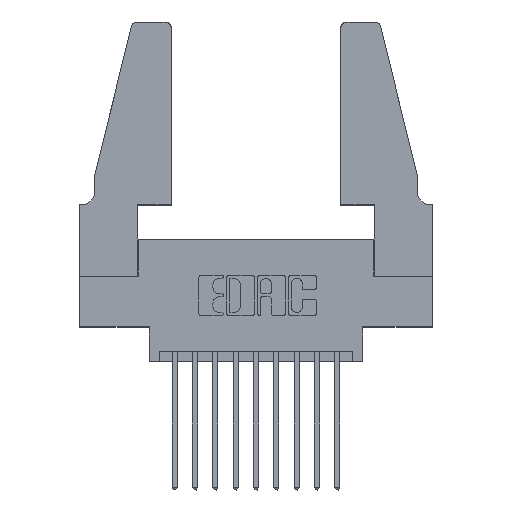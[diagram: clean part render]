
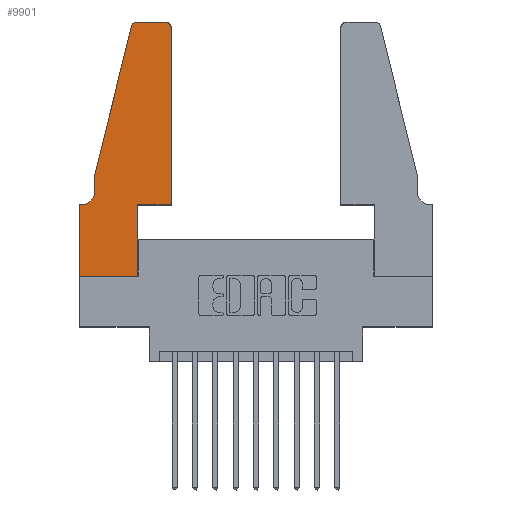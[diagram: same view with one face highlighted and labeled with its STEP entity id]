
A CAD part, top view. The second image highlights one B-rep face of the part: STEP entity #9901.
In plain terms, the highlighted planar face has unit normal (0, 0, 1).
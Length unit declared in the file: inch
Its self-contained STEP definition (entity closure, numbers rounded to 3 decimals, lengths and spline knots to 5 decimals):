
#49 = EDGE_CURVE ( 'NONE', #7841, #9602, #7819, .T. ) ;
#59 = DIRECTION ( 'NONE',  ( -1., 0., 0. ) ) ;
#118 = CARTESIAN_POINT ( 'NONE',  ( 0.2865, 0.35, 0.37 ) ) ;
#161 = DIRECTION ( 'NONE',  ( 0., 1., 0. ) ) ;
#573 = CARTESIAN_POINT ( 'NONE',  ( 0.2865, 0.35, 0.37 ) ) ;
#742 = ORIENTED_EDGE ( 'NONE', *, *, #4941, .T. ) ;
#955 = LINE ( 'NONE', #10663, #5234 ) ;
#1137 = DIRECTION ( 'NONE',  ( -1., 0., 0. ) ) ;
#1198 = VERTEX_POINT ( 'NONE', #6475 ) ;
#1309 = CARTESIAN_POINT ( 'NONE',  ( 0.0755, 0.5, 0.37 ) ) ;
#1310 = DIRECTION ( 'NONE',  ( -1., 0., 0. ) ) ;
#1605 = EDGE_LOOP ( 'NONE', ( #12128, #742, #8746, #7917, #6020, #7271, #11138, #9298, #1610, #8991, #12434, #9938 ) ) ;
#1610 = ORIENTED_EDGE ( 'NONE', *, *, #8606, .T. ) ;
#1633 = DIRECTION ( 'NONE',  ( 1., 0., 0. ) ) ;
#2351 = CARTESIAN_POINT ( 'NONE',  ( 0.4205, 1.22, 0.37 ) ) ;
#3048 = LINE ( 'NONE', #11679, #7726 ) ;
#3116 = EDGE_CURVE ( 'NONE', #10071, #5017, #7274, .T. ) ;
#3377 = CARTESIAN_POINT ( 'NONE',  ( 0.0055, 0.42, 0.37 ) ) ;
#3413 = CARTESIAN_POINT ( 'NONE',  ( 0.284, 1.22, 0.37 ) ) ;
#3847 = CARTESIAN_POINT ( 'NONE',  ( 0.4205, 1.25, 0.37 ) ) ;
#4272 = DIRECTION ( 'NONE',  ( 0., -1., 0. ) ) ;
#4383 = DIRECTION ( 'NONE',  ( 0., -1., 0. ) ) ;
#4542 = EDGE_CURVE ( 'NONE', #12759, #10071, #8392, .T. ) ;
#4570 = DIRECTION ( 'NONE',  ( 1., 0., 0. ) ) ;
#4941 = EDGE_CURVE ( 'NONE', #1198, #10855, #8474, .T. ) ;
#4995 = CARTESIAN_POINT ( 'NONE',  ( 0.4505, 1.22, 0.37 ) ) ;
#5017 = VERTEX_POINT ( 'NONE', #11174 ) ;
#5051 = VECTOR ( 'NONE', #4383, 39.37008 ) ;
#5080 = DIRECTION ( 'NONE',  ( 1., 0., 0. ) ) ;
#5096 = VERTEX_POINT ( 'NONE', #13667 ) ;
#5234 = VECTOR ( 'NONE', #4272, 39.37008 ) ;
#5282 = CARTESIAN_POINT ( 'NONE',  ( 0.0755, 0.35, 0.37 ) ) ;
#5436 = AXIS2_PLACEMENT_3D ( 'NONE', #3413, #5685, #6741 ) ;
#5554 = AXIS2_PLACEMENT_3D ( 'NONE', #11178, #7035, #1633 ) ;
#5685 = DIRECTION ( 'NONE',  ( 0., 0., 1. ) ) ;
#5698 = VECTOR ( 'NONE', #161, 39.37008 ) ;
#6020 = ORIENTED_EDGE ( 'NONE', *, *, #4542, .T. ) ;
#6046 = VERTEX_POINT ( 'NONE', #8072 ) ;
#6053 = LINE ( 'NONE', #118, #5698 ) ;
#6338 = FACE_OUTER_BOUND ( 'NONE', #1605, .T. ) ;
#6475 = CARTESIAN_POINT ( 'NONE',  ( 0.284, 1.25, 0.37 ) ) ;
#6741 = DIRECTION ( 'NONE',  ( 1., 0., 0. ) ) ;
#6918 = VECTOR ( 'NONE', #7499, 39.37008 ) ;
#6952 = EDGE_CURVE ( 'NONE', #6046, #5096, #13807, .T. ) ;
#7035 = DIRECTION ( 'NONE',  ( 0., 0., 1. ) ) ;
#7271 = ORIENTED_EDGE ( 'NONE', *, *, #3116, .T. ) ;
#7274 = LINE ( 'NONE', #5282, #12598 ) ;
#7499 = DIRECTION ( 'NONE',  ( -0.239, -0.971, 0. ) ) ;
#7674 = CARTESIAN_POINT ( 'NONE',  ( 0.0755, 0.42, 0.37 ) ) ;
#7726 = VECTOR ( 'NONE', #59, 39.37008 ) ;
#7819 = CIRCLE ( 'NONE', #7831, 0.03 ) ;
#7831 = AXIS2_PLACEMENT_3D ( 'NONE', #2351, #11991, #4570 ) ;
#7841 = VERTEX_POINT ( 'NONE', #4995 ) ;
#7917 = ORIENTED_EDGE ( 'NONE', *, *, #11423, .T. ) ;
#8072 = CARTESIAN_POINT ( 'NONE',  ( 0., 0., 0.37 ) ) ;
#8118 = VECTOR ( 'NONE', #12546, 39.37008 ) ;
#8348 = VECTOR ( 'NONE', #5080, 39.37008 ) ;
#8385 = EDGE_CURVE ( 'NONE', #8601, #7841, #9073, .T. ) ;
#8392 = CIRCLE ( 'NONE', #10286, 0.07 ) ;
#8396 = DIRECTION ( 'NONE',  ( 0., 1., 0. ) ) ;
#8474 = CIRCLE ( 'NONE', #5436, 0.03 ) ;
#8567 = EDGE_CURVE ( 'NONE', #5017, #6046, #12408, .T. ) ;
#8601 = VERTEX_POINT ( 'NONE', #10777 ) ;
#8606 = EDGE_CURVE ( 'NONE', #5096, #9912, #6053, .T. ) ;
#8746 = ORIENTED_EDGE ( 'NONE', *, *, #12713, .T. ) ;
#8991 = ORIENTED_EDGE ( 'NONE', *, *, #11323, .T. ) ;
#9073 = LINE ( 'NONE', #13731, #10068 ) ;
#9298 = ORIENTED_EDGE ( 'NONE', *, *, #6952, .T. ) ;
#9541 = CARTESIAN_POINT ( 'NONE',  ( 0.0755, 0.5, 0.37 ) ) ;
#9602 = VERTEX_POINT ( 'NONE', #3847 ) ;
#9901 = ADVANCED_FACE ( 'NONE', ( #6338 ), #13437, .T. ) ;
#9912 = VERTEX_POINT ( 'NONE', #573 ) ;
#9938 = ORIENTED_EDGE ( 'NONE', *, *, #49, .T. ) ;
#10068 = VECTOR ( 'NONE', #8396, 39.37008 ) ;
#10071 = VERTEX_POINT ( 'NONE', #10159 ) ;
#10159 = CARTESIAN_POINT ( 'NONE',  ( 0.0055, 0.35, 0.37 ) ) ;
#10286 = AXIS2_PLACEMENT_3D ( 'NONE', #3377, #10845, #1310 ) ;
#10663 = CARTESIAN_POINT ( 'NONE',  ( 0.0755, 0.5, 0.37 ) ) ;
#10777 = CARTESIAN_POINT ( 'NONE',  ( 0.4505, 0.35, 0.37 ) ) ;
#10845 = DIRECTION ( 'NONE',  ( 0., 0., -1. ) ) ;
#10855 = VERTEX_POINT ( 'NONE', #13633 ) ;
#11138 = ORIENTED_EDGE ( 'NONE', *, *, #8567, .T. ) ;
#11174 = CARTESIAN_POINT ( 'NONE',  ( 0., 0.35, 0.37 ) ) ;
#11178 = CARTESIAN_POINT ( 'NONE',  ( 0., 0.35, 0.37 ) ) ;
#11323 = EDGE_CURVE ( 'NONE', #9912, #8601, #12502, .T. ) ;
#11423 = EDGE_CURVE ( 'NONE', #11981, #12759, #955, .T. ) ;
#11430 = LINE ( 'NONE', #9541, #6918 ) ;
#11679 = CARTESIAN_POINT ( 'NONE',  ( 0.2605, 1.25, 0.37 ) ) ;
#11807 = CARTESIAN_POINT ( 'NONE',  ( 0., 0., 0.37 ) ) ;
#11981 = VERTEX_POINT ( 'NONE', #1309 ) ;
#11991 = DIRECTION ( 'NONE',  ( 0., 0., 1. ) ) ;
#12128 = ORIENTED_EDGE ( 'NONE', *, *, #13525, .T. ) ;
#12408 = LINE ( 'NONE', #11807, #5051 ) ;
#12434 = ORIENTED_EDGE ( 'NONE', *, *, #8385, .T. ) ;
#12502 = LINE ( 'NONE', #13699, #8348 ) ;
#12546 = DIRECTION ( 'NONE',  ( 1., 0., 0. ) ) ;
#12590 = CARTESIAN_POINT ( 'NONE',  ( 0., 0., 0.37 ) ) ;
#12598 = VECTOR ( 'NONE', #1137, 39.37008 ) ;
#12713 = EDGE_CURVE ( 'NONE', #10855, #11981, #11430, .T. ) ;
#12759 = VERTEX_POINT ( 'NONE', #7674 ) ;
#13437 = PLANE ( 'NONE',  #5554 ) ;
#13525 = EDGE_CURVE ( 'NONE', #9602, #1198, #3048, .T. ) ;
#13633 = CARTESIAN_POINT ( 'NONE',  ( 0.25487, 1.22718, 0.37 ) ) ;
#13667 = CARTESIAN_POINT ( 'NONE',  ( 0.2865, 0., 0.37 ) ) ;
#13699 = CARTESIAN_POINT ( 'NONE',  ( 0.4505, 0.35, 0.37 ) ) ;
#13731 = CARTESIAN_POINT ( 'NONE',  ( 0.4505, 0.35, 0.37 ) ) ;
#13807 = LINE ( 'NONE', #12590, #8118 ) ;
